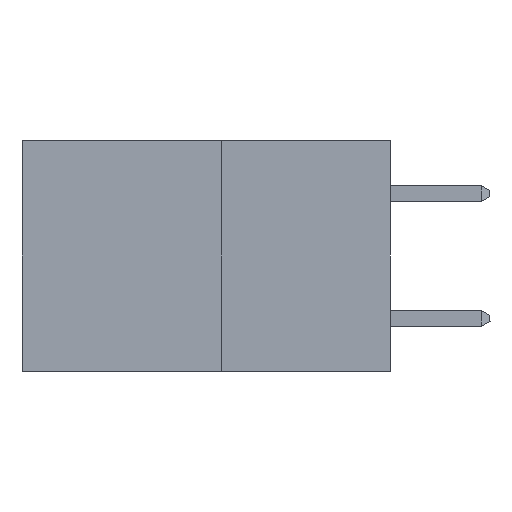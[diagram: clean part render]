
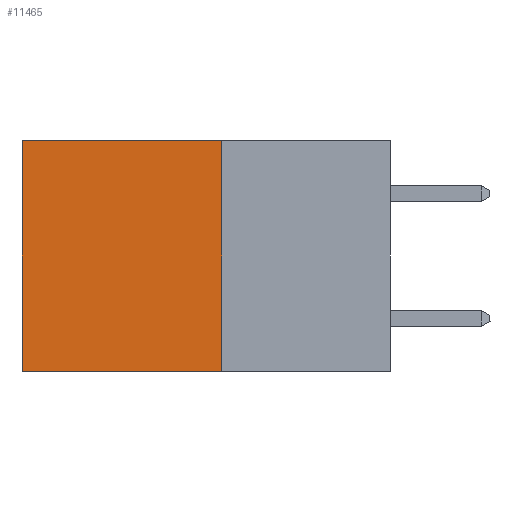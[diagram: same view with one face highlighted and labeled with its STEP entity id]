
A CAD part, left-side view. The second image highlights one B-rep face of the part: STEP entity #11465.
In plain terms, the highlighted planar face has unit normal (-1, 0, 0).
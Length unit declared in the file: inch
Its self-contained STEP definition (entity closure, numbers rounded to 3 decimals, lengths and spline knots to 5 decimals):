
#925 = LINE ( 'NONE', #1181, #10250 ) ;
#1181 = CARTESIAN_POINT ( 'NONE',  ( 0.277, 0.59, -0.37 ) ) ;
#1259 = PLANE ( 'NONE',  #12940 ) ;
#1831 = EDGE_CURVE ( 'NONE', #13622, #12835, #14381, .T. ) ;
#1891 = DIRECTION ( 'NONE',  ( 0., 0., -1. ) ) ;
#2431 = DIRECTION ( 'NONE',  ( 1., 0., 0. ) ) ;
#2571 = VECTOR ( 'NONE', #8278, 39.37008 ) ;
#2834 = DIRECTION ( 'NONE',  ( 0., 1., 0. ) ) ;
#3023 = CARTESIAN_POINT ( 'NONE',  ( 0.277, 0.59, 0. ) ) ;
#3260 = ORIENTED_EDGE ( 'NONE', *, *, #7287, .T. ) ;
#3441 = ORIENTED_EDGE ( 'NONE', *, *, #9665, .F. ) ;
#5573 = VERTEX_POINT ( 'NONE', #3023 ) ;
#5884 = EDGE_CURVE ( 'NONE', #13622, #5573, #8436, .T. ) ;
#7090 = CARTESIAN_POINT ( 'NONE',  ( 0.277, 0.27, 0. ) ) ;
#7287 = EDGE_CURVE ( 'NONE', #5573, #14228, #925, .T. ) ;
#8268 = CARTESIAN_POINT ( 'NONE',  ( 0.277, 0.27, -0.37 ) ) ;
#8278 = DIRECTION ( 'NONE',  ( 0., 1., 0. ) ) ;
#8436 = LINE ( 'NONE', #7090, #2571 ) ;
#8665 = CARTESIAN_POINT ( 'NONE',  ( 0.277, 0.27, -0.37 ) ) ;
#8939 = VECTOR ( 'NONE', #1891, 39.37008 ) ;
#9355 = DIRECTION ( 'NONE',  ( 0., 0., -1. ) ) ;
#9665 = EDGE_CURVE ( 'NONE', #12835, #14228, #11883, .T. ) ;
#10250 = VECTOR ( 'NONE', #9355, 39.37008 ) ;
#10619 = DIRECTION ( 'NONE',  ( 0., 0., -1. ) ) ;
#11465 = ADVANCED_FACE ( 'NONE', ( #11826 ), #1259, .F. ) ;
#11826 = FACE_OUTER_BOUND ( 'NONE', #14824, .T. ) ;
#11883 = LINE ( 'NONE', #8665, #14226 ) ;
#12835 = VERTEX_POINT ( 'NONE', #14136 ) ;
#12940 = AXIS2_PLACEMENT_3D ( 'NONE', #8268, #2431, #10619 ) ;
#13021 = CARTESIAN_POINT ( 'NONE',  ( 0.277, 0.27, 0. ) ) ;
#13598 = ORIENTED_EDGE ( 'NONE', *, *, #1831, .F. ) ;
#13622 = VERTEX_POINT ( 'NONE', #13021 ) ;
#14136 = CARTESIAN_POINT ( 'NONE',  ( 0.277, 0.27, -0.37 ) ) ;
#14226 = VECTOR ( 'NONE', #2834, 39.37008 ) ;
#14228 = VERTEX_POINT ( 'NONE', #14735 ) ;
#14381 = LINE ( 'NONE', #14725, #8939 ) ;
#14460 = ORIENTED_EDGE ( 'NONE', *, *, #5884, .T. ) ;
#14725 = CARTESIAN_POINT ( 'NONE',  ( 0.277, 0.27, -0.37 ) ) ;
#14735 = CARTESIAN_POINT ( 'NONE',  ( 0.277, 0.59, -0.37 ) ) ;
#14824 = EDGE_LOOP ( 'NONE', ( #3260, #3441, #13598, #14460 ) ) ;
